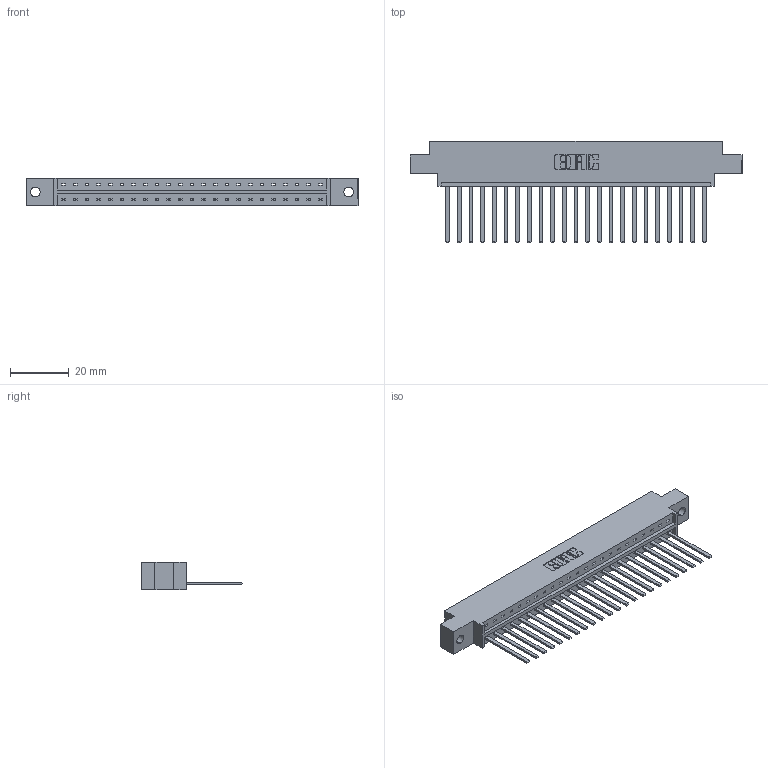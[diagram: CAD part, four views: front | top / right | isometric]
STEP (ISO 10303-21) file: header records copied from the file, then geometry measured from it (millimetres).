
FILE_DESCRIPTION (( 'STEP AP203' ), '1' );
FILE_NAME ('833-023-544-602.STEP', '2020-06-01T19:34:15', ( '' ), ( '' ), 'SwSTEP 2.0', 'SolidWorks 2020', '' );
FILE_SCHEMA (( 'CONFIG_CONTROL_DESIGN' ));
Length unit declared in the file: inch
Products named in the file (3): 345-292-001_345-293-144; 833-023-544-602; 833 Part_Offset - .128 Dia
Assembly tree (24 placements, depth 2):
  833-023-544-602
    833 Part_Offset - .128 Dia
    345-292-001_345-293-144  x23
Bounding box: 112.67 x 34.3 x 9.4 mm (x, y, z)
Volume: 11176.7 mm3; surface area: 12760.5 mm2
Topology: 24 solids, 24 shells, 1314 faces, 3957 edges, 2606 vertices
Faces by surface type: plane 948, cylinder 366
Entity records: 16469 total; most frequent: CARTESIAN_POINT 2851, ORIENTED_EDGE 2810, DIRECTION 2439, EDGE_CURVE 1405, LINE 1281, VECTOR 1281, VERTEX_POINT 934, AXIS2_PLACEMENT_3D 579
